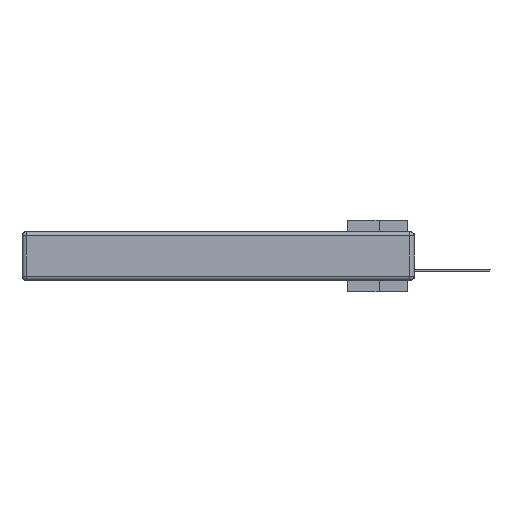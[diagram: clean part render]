
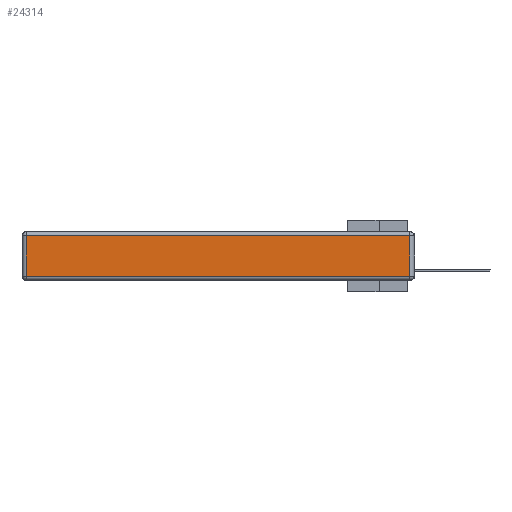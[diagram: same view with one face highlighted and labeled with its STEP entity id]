
A CAD part, left-side view. The second image highlights one B-rep face of the part: STEP entity #24314.
In plain terms, the highlighted planar face has unit normal (-1, 0, 0).
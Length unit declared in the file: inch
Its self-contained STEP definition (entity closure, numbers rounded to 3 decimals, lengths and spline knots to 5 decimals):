
#228 = ORIENTED_EDGE ( 'NONE', *, *, #27898, .T. ) ;
#1072 = CARTESIAN_POINT ( 'NONE',  ( 0., 0., -0.313 ) ) ;
#3221 = DIRECTION ( 'NONE',  ( -1., 0., 0. ) ) ;
#5100 = VECTOR ( 'NONE', #10326, 39.37008 ) ;
#5396 = CARTESIAN_POINT ( 'NONE',  ( 0., 2.72, -0.313 ) ) ;
#5819 = DIRECTION ( 'NONE',  ( 0., -1., 0. ) ) ;
#6379 = CARTESIAN_POINT ( 'NONE',  ( 0., 2.72, -0.343 ) ) ;
#7384 = DIRECTION ( 'NONE',  ( 0., 1., 0. ) ) ;
#7738 = CARTESIAN_POINT ( 'NONE',  ( 0., 0.03, -0.313 ) ) ;
#9575 = EDGE_CURVE ( 'NONE', #12444, #12045, #21366, .T. ) ;
#10326 = DIRECTION ( 'NONE',  ( 0., 0., -1. ) ) ;
#10815 = VECTOR ( 'NONE', #28145, 39.37008 ) ;
#12045 = VERTEX_POINT ( 'NONE', #27414 ) ;
#12270 = EDGE_LOOP ( 'NONE', ( #18010, #22148, #18349, #228 ) ) ;
#12444 = VERTEX_POINT ( 'NONE', #7738 ) ;
#12474 = VECTOR ( 'NONE', #7384, 39.37008 ) ;
#14629 = EDGE_CURVE ( 'NONE', #12045, #23360, #23140, .T. ) ;
#15785 = LINE ( 'NONE', #6379, #5100 ) ;
#16203 = CARTESIAN_POINT ( 'NONE',  ( 0., 2.75, -0.03 ) ) ;
#16630 = PLANE ( 'NONE',  #22388 ) ;
#18010 = ORIENTED_EDGE ( 'NONE', *, *, #26443, .T. ) ;
#18349 = ORIENTED_EDGE ( 'NONE', *, *, #14629, .T. ) ;
#18700 = FACE_OUTER_BOUND ( 'NONE', #12270, .T. ) ;
#19148 = CARTESIAN_POINT ( 'NONE',  ( 0., 0.03, -0.343 ) ) ;
#21366 = LINE ( 'NONE', #19148, #10815 ) ;
#21961 = CARTESIAN_POINT ( 'NONE',  ( 0., 2.72, -0.03 ) ) ;
#22030 = VECTOR ( 'NONE', #5819, 39.37008 ) ;
#22148 = ORIENTED_EDGE ( 'NONE', *, *, #9575, .T. ) ;
#22388 = AXIS2_PLACEMENT_3D ( 'NONE', #27412, #3221, #25633 ) ;
#23140 = LINE ( 'NONE', #16203, #12474 ) ;
#23360 = VERTEX_POINT ( 'NONE', #21961 ) ;
#24314 = ADVANCED_FACE ( 'NONE', ( #18700 ), #16630, .T. ) ;
#25633 = DIRECTION ( 'NONE',  ( 0., 0., 1. ) ) ;
#26443 = EDGE_CURVE ( 'NONE', #28538, #12444, #28519, .T. ) ;
#27412 = CARTESIAN_POINT ( 'NONE',  ( 0., 0., -0.343 ) ) ;
#27414 = CARTESIAN_POINT ( 'NONE',  ( 0., 0.03, -0.03 ) ) ;
#27898 = EDGE_CURVE ( 'NONE', #23360, #28538, #15785, .T. ) ;
#28145 = DIRECTION ( 'NONE',  ( 0., 0., 1. ) ) ;
#28519 = LINE ( 'NONE', #1072, #22030 ) ;
#28538 = VERTEX_POINT ( 'NONE', #5396 ) ;
